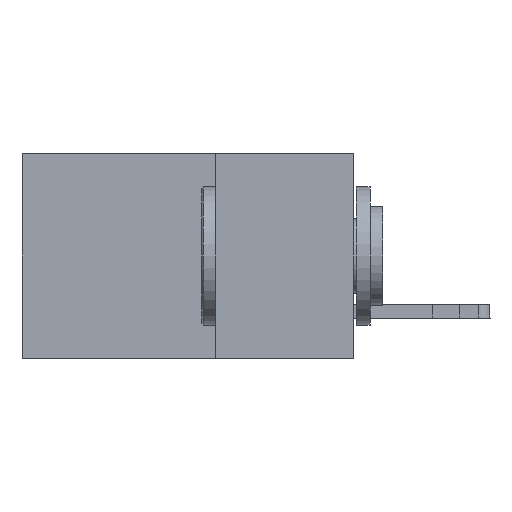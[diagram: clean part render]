
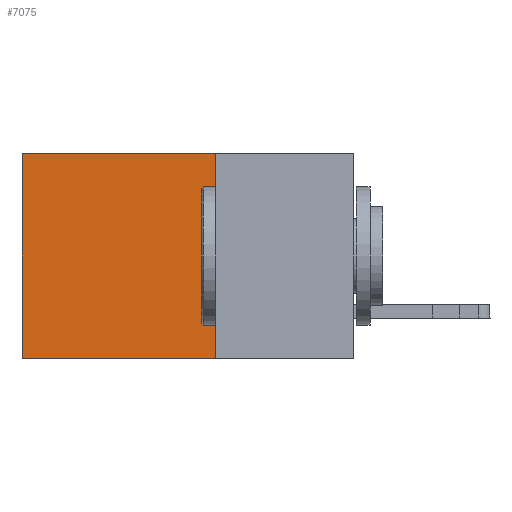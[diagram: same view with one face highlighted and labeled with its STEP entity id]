
A CAD part, left-side view. The second image highlights one B-rep face of the part: STEP entity #7075.
In plain terms, the highlighted planar face has unit normal (-1, 0, 0).
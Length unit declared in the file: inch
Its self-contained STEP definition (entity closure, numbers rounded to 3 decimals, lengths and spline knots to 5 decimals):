
#1111 = VECTOR ( 'NONE', #32084, 39.37008 ) ;
#2290 = EDGE_CURVE ( 'NONE', #26490, #30313, #11942, .T. ) ;
#3022 = CARTESIAN_POINT ( 'NONE',  ( 0.2875, 0.25, -0.37 ) ) ;
#3482 = ORIENTED_EDGE ( 'NONE', *, *, #27545, .F. ) ;
#4054 = EDGE_CURVE ( 'NONE', #26490, #36931, #20299, .T. ) ;
#4407 = DIRECTION ( 'NONE',  ( 1., 0., 0. ) ) ;
#6501 = DIRECTION ( 'NONE',  ( 0., 1., 0. ) ) ;
#7075 = ADVANCED_FACE ( 'NONE', ( #25200 ), #35596, .F. ) ;
#7778 = CARTESIAN_POINT ( 'NONE',  ( 0.2875, 0.25, 0. ) ) ;
#9808 = CARTESIAN_POINT ( 'NONE',  ( 0.2875, 0.6, 0. ) ) ;
#10486 = CARTESIAN_POINT ( 'NONE',  ( 0.2875, 0.25, 0. ) ) ;
#11942 = LINE ( 'NONE', #24747, #24320 ) ;
#15709 = ORIENTED_EDGE ( 'NONE', *, *, #29129, .T. ) ;
#16331 = CARTESIAN_POINT ( 'NONE',  ( 0.2875, 0.6, 0. ) ) ;
#18007 = CARTESIAN_POINT ( 'NONE',  ( 0.2875, 0.6, -0.37 ) ) ;
#18339 = EDGE_LOOP ( 'NONE', ( #15709, #3482, #39006, #37804 ) ) ;
#20299 = LINE ( 'NONE', #7778, #1111 ) ;
#20638 = LINE ( 'NONE', #3022, #31079 ) ;
#21576 = CARTESIAN_POINT ( 'NONE',  ( 0.2875, 0.25, -0.37 ) ) ;
#24320 = VECTOR ( 'NONE', #6501, 39.37008 ) ;
#24747 = CARTESIAN_POINT ( 'NONE',  ( 0.2875, 0.25, 0. ) ) ;
#25200 = FACE_OUTER_BOUND ( 'NONE', #18339, .T. ) ;
#26490 = VERTEX_POINT ( 'NONE', #10486 ) ;
#27545 = EDGE_CURVE ( 'NONE', #36931, #37578, #20638, .T. ) ;
#28392 = AXIS2_PLACEMENT_3D ( 'NONE', #33559, #4407, #34975 ) ;
#29129 = EDGE_CURVE ( 'NONE', #30313, #37578, #39164, .T. ) ;
#30313 = VERTEX_POINT ( 'NONE', #16331 ) ;
#30498 = DIRECTION ( 'NONE',  ( 0., 1., 0. ) ) ;
#31079 = VECTOR ( 'NONE', #30498, 39.37008 ) ;
#31153 = DIRECTION ( 'NONE',  ( 0., 0., -1. ) ) ;
#32084 = DIRECTION ( 'NONE',  ( 0., 0., -1. ) ) ;
#33559 = CARTESIAN_POINT ( 'NONE',  ( 0.2875, 0.25, 0. ) ) ;
#34975 = DIRECTION ( 'NONE',  ( 0., 0., -1. ) ) ;
#35596 = PLANE ( 'NONE',  #28392 ) ;
#36931 = VERTEX_POINT ( 'NONE', #21576 ) ;
#37176 = VECTOR ( 'NONE', #31153, 39.37008 ) ;
#37578 = VERTEX_POINT ( 'NONE', #18007 ) ;
#37804 = ORIENTED_EDGE ( 'NONE', *, *, #2290, .T. ) ;
#39006 = ORIENTED_EDGE ( 'NONE', *, *, #4054, .F. ) ;
#39164 = LINE ( 'NONE', #9808, #37176 ) ;
